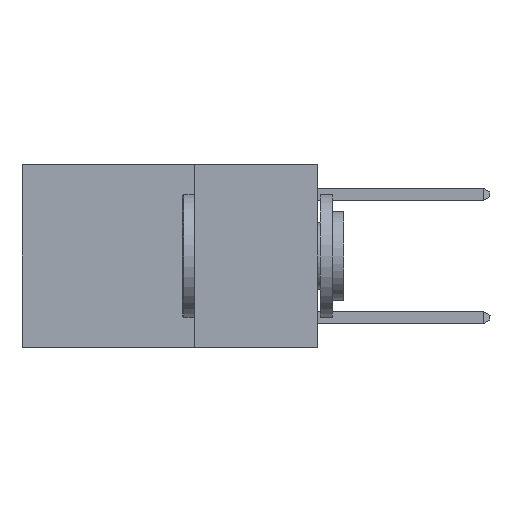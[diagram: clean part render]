
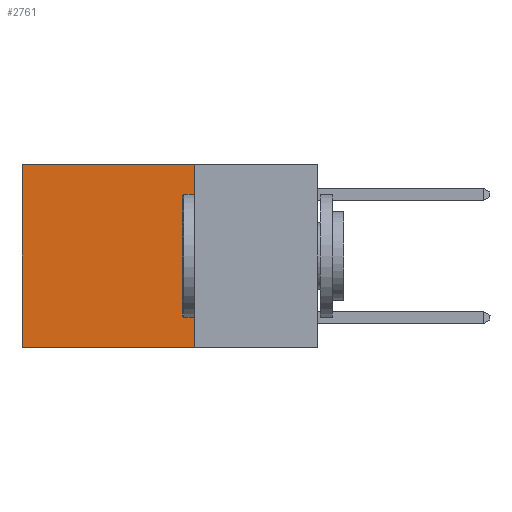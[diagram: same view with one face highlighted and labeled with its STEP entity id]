
A CAD part, left-side view. The second image highlights one B-rep face of the part: STEP entity #2761.
In plain terms, the highlighted planar face has unit normal (-1, 0, 0).
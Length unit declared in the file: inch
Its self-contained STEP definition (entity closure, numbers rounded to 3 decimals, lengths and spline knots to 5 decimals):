
#115 = VERTEX_POINT ( 'NONE', #7478 ) ;
#1465 = EDGE_CURVE ( 'NONE', #4186, #20103, #22226, .T. ) ;
#1963 = ORIENTED_EDGE ( 'NONE', *, *, #11408, .T. ) ;
#2761 = ADVANCED_FACE ( 'NONE', ( #10119 ), #6356, .F. ) ;
#2803 = VECTOR ( 'NONE', #10631, 39.37008 ) ;
#2854 = ORIENTED_EDGE ( 'NONE', *, *, #4102, .F. ) ;
#3950 = EDGE_LOOP ( 'NONE', ( #1963, #7299, #2854, #8920 ) ) ;
#4102 = EDGE_CURVE ( 'NONE', #6116, #4186, #8990, .T. ) ;
#4186 = VERTEX_POINT ( 'NONE', #12867 ) ;
#6116 = VERTEX_POINT ( 'NONE', #16196 ) ;
#6356 = PLANE ( 'NONE',  #21825 ) ;
#7299 = ORIENTED_EDGE ( 'NONE', *, *, #1465, .F. ) ;
#7478 = CARTESIAN_POINT ( 'NONE',  ( 0.2625, 0.6, 0. ) ) ;
#7811 = LINE ( 'NONE', #8949, #2803 ) ;
#8920 = ORIENTED_EDGE ( 'NONE', *, *, #16462, .T. ) ;
#8949 = CARTESIAN_POINT ( 'NONE',  ( 0.2625, 0.25, 0. ) ) ;
#8990 = LINE ( 'NONE', #22309, #9518 ) ;
#9160 = VECTOR ( 'NONE', #13025, 39.37008 ) ;
#9518 = VECTOR ( 'NONE', #10911, 39.37008 ) ;
#10119 = FACE_OUTER_BOUND ( 'NONE', #3950, .T. ) ;
#10631 = DIRECTION ( 'NONE',  ( 0., 1., 0. ) ) ;
#10911 = DIRECTION ( 'NONE',  ( 0., 0., -1. ) ) ;
#11035 = DIRECTION ( 'NONE',  ( 0., 0., -1. ) ) ;
#11408 = EDGE_CURVE ( 'NONE', #115, #20103, #21378, .T. ) ;
#11591 = DIRECTION ( 'NONE',  ( 0., 0., -1. ) ) ;
#12867 = CARTESIAN_POINT ( 'NONE',  ( 0.2625, 0.25, -0.37 ) ) ;
#13025 = DIRECTION ( 'NONE',  ( 0., 1., 0. ) ) ;
#13095 = CARTESIAN_POINT ( 'NONE',  ( 0.2625, 0.25, -0.37 ) ) ;
#13252 = CARTESIAN_POINT ( 'NONE',  ( 0.2625, 0.25, 0. ) ) ;
#14063 = CARTESIAN_POINT ( 'NONE',  ( 0.2625, 0.6, -0.37 ) ) ;
#14429 = CARTESIAN_POINT ( 'NONE',  ( 0.2625, 0.6, 0. ) ) ;
#16196 = CARTESIAN_POINT ( 'NONE',  ( 0.2625, 0.25, 0. ) ) ;
#16462 = EDGE_CURVE ( 'NONE', #6116, #115, #7811, .T. ) ;
#17151 = VECTOR ( 'NONE', #11035, 39.37008 ) ;
#20103 = VERTEX_POINT ( 'NONE', #14063 ) ;
#21335 = DIRECTION ( 'NONE',  ( 1., 0., 0. ) ) ;
#21378 = LINE ( 'NONE', #14429, #17151 ) ;
#21825 = AXIS2_PLACEMENT_3D ( 'NONE', #13252, #21335, #11591 ) ;
#22226 = LINE ( 'NONE', #13095, #9160 ) ;
#22309 = CARTESIAN_POINT ( 'NONE',  ( 0.2625, 0.25, 0. ) ) ;
